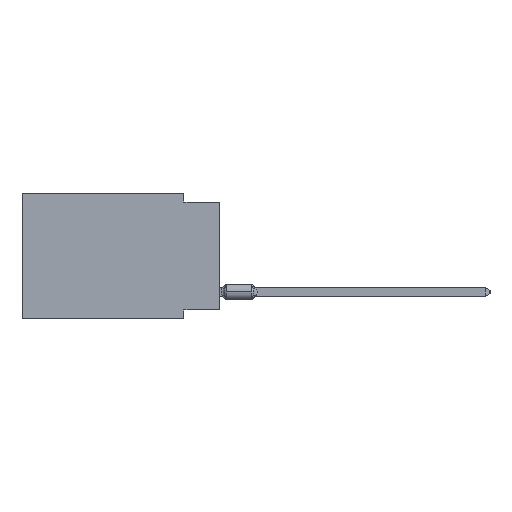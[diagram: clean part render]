
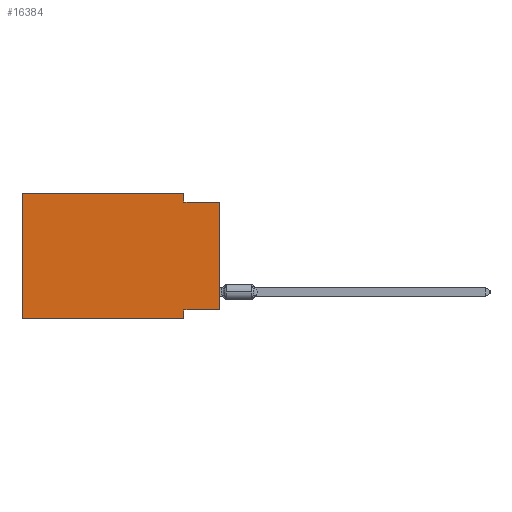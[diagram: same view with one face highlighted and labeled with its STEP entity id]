
A CAD part, left-side view. The second image highlights one B-rep face of the part: STEP entity #16384.
In plain terms, the highlighted planar face has unit normal (-1, 0, 0).
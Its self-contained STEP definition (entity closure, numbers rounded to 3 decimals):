
#839 = VECTOR ( 'NONE', #49337, 1000. ) ;
#1017 = EDGE_LOOP ( 'NONE', ( #6531, #81549, #19849, #11242, #34195, #32666, #28479, #76534 ) ) ;
#1175 = LINE ( 'NONE', #21528, #16416 ) ;
#3059 = VERTEX_POINT ( 'NONE', #69449 ) ;
#6531 = ORIENTED_EDGE ( 'NONE', *, *, #48440, .T. ) ;
#8270 = DIRECTION ( 'NONE',  ( 0., -1., 0. ) ) ;
#9687 = CARTESIAN_POINT ( 'NONE',  ( 0., 13.97, 0. ) ) ;
#11111 = VECTOR ( 'NONE', #27631, 1000. ) ;
#11242 = ORIENTED_EDGE ( 'NONE', *, *, #17975, .F. ) ;
#13111 = CARTESIAN_POINT ( 'NONE',  ( 0., 0., -0.635 ) ) ;
#15135 = LINE ( 'NONE', #42099, #28464 ) ;
#15972 = CARTESIAN_POINT ( 'NONE',  ( 0., 2.54, -8.89 ) ) ;
#16268 = CARTESIAN_POINT ( 'NONE',  ( 0., 13.97, -8.89 ) ) ;
#16384 = ADVANCED_FACE ( 'NONE', ( #47824 ), #26617, .F. ) ;
#16416 = VECTOR ( 'NONE', #8270, 1000. ) ;
#17975 = EDGE_CURVE ( 'NONE', #46248, #80970, #15135, .T. ) ;
#19849 = ORIENTED_EDGE ( 'NONE', *, *, #78689, .F. ) ;
#20078 = CARTESIAN_POINT ( 'NONE',  ( 0., 2.54, 0. ) ) ;
#21528 = CARTESIAN_POINT ( 'NONE',  ( 0., 0., -0.635 ) ) ;
#22798 = CARTESIAN_POINT ( 'NONE',  ( 0., 13.97, -8.89 ) ) ;
#24071 = EDGE_CURVE ( 'NONE', #3059, #77037, #1175, .T. ) ;
#25770 = DIRECTION ( 'NONE',  ( 0., 0., 1. ) ) ;
#26617 = PLANE ( 'NONE',  #81878 ) ;
#27631 = DIRECTION ( 'NONE',  ( 0., 0., -1. ) ) ;
#28464 = VECTOR ( 'NONE', #55354, 1000. ) ;
#28479 = ORIENTED_EDGE ( 'NONE', *, *, #41826, .F. ) ;
#29156 = DIRECTION ( 'NONE',  ( 0., 1., 0. ) ) ;
#31074 = VECTOR ( 'NONE', #64900, 1000. ) ;
#32666 = ORIENTED_EDGE ( 'NONE', *, *, #60527, .T. ) ;
#34195 = ORIENTED_EDGE ( 'NONE', *, *, #61290, .F. ) ;
#34704 = CARTESIAN_POINT ( 'NONE',  ( 0., 2.54, -8.89 ) ) ;
#36208 = CARTESIAN_POINT ( 'NONE',  ( 0., 0., -8.255 ) ) ;
#36924 = LINE ( 'NONE', #22798, #839 ) ;
#37943 = CARTESIAN_POINT ( 'NONE',  ( 0., 2.54, 0. ) ) ;
#39178 = VECTOR ( 'NONE', #78908, 1000. ) ;
#40384 = CARTESIAN_POINT ( 'NONE',  ( 0., 0., -8.255 ) ) ;
#40432 = VECTOR ( 'NONE', #25770, 1000. ) ;
#41415 = CARTESIAN_POINT ( 'NONE',  ( 0., 2.54, -8.255 ) ) ;
#41826 = EDGE_CURVE ( 'NONE', #45247, #82828, #55047, .T. ) ;
#42099 = CARTESIAN_POINT ( 'NONE',  ( 0., 13.97, 0. ) ) ;
#44569 = LINE ( 'NONE', #37943, #31074 ) ;
#45247 = VERTEX_POINT ( 'NONE', #41415 ) ;
#46248 = VERTEX_POINT ( 'NONE', #9687 ) ;
#47824 = FACE_OUTER_BOUND ( 'NONE', #1017, .T. ) ;
#48440 = EDGE_CURVE ( 'NONE', #69226, #77037, #78864, .T. ) ;
#49337 = DIRECTION ( 'NONE',  ( 0., -1., 0. ) ) ;
#52391 = VECTOR ( 'NONE', #29156, 1000. ) ;
#52798 = LINE ( 'NONE', #58995, #39178 ) ;
#54018 = CARTESIAN_POINT ( 'NONE',  ( 0., 13.97, 0. ) ) ;
#55047 = LINE ( 'NONE', #34704, #11111 ) ;
#55354 = DIRECTION ( 'NONE',  ( 0., -1., 0. ) ) ;
#58995 = CARTESIAN_POINT ( 'NONE',  ( 0., 13.97, 0. ) ) ;
#60527 = EDGE_CURVE ( 'NONE', #64380, #82828, #36924, .T. ) ;
#61290 = EDGE_CURVE ( 'NONE', #64380, #46248, #52798, .T. ) ;
#64380 = VERTEX_POINT ( 'NONE', #16268 ) ;
#64900 = DIRECTION ( 'NONE',  ( 0., 0., -1. ) ) ;
#69226 = VERTEX_POINT ( 'NONE', #40384 ) ;
#69449 = CARTESIAN_POINT ( 'NONE',  ( 0., 2.54, -0.635 ) ) ;
#70259 = LINE ( 'NONE', #36208, #52391 ) ;
#72221 = CARTESIAN_POINT ( 'NONE',  ( 0., 0., 0. ) ) ;
#73939 = DIRECTION ( 'NONE',  ( 0., 0., -1. ) ) ;
#76534 = ORIENTED_EDGE ( 'NONE', *, *, #79693, .F. ) ;
#77037 = VERTEX_POINT ( 'NONE', #13111 ) ;
#78689 = EDGE_CURVE ( 'NONE', #80970, #3059, #44569, .T. ) ;
#78864 = LINE ( 'NONE', #72221, #40432 ) ;
#78908 = DIRECTION ( 'NONE',  ( 0., 0., 1. ) ) ;
#79693 = EDGE_CURVE ( 'NONE', #69226, #45247, #70259, .T. ) ;
#80970 = VERTEX_POINT ( 'NONE', #20078 ) ;
#81549 = ORIENTED_EDGE ( 'NONE', *, *, #24071, .F. ) ;
#81878 = AXIS2_PLACEMENT_3D ( 'NONE', #54018, #86793, #73939 ) ;
#82828 = VERTEX_POINT ( 'NONE', #15972 ) ;
#86793 = DIRECTION ( 'NONE',  ( 1., 0., 0. ) ) ;
